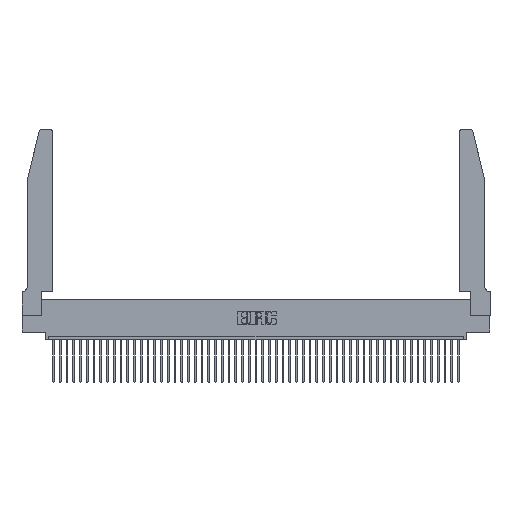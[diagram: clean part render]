
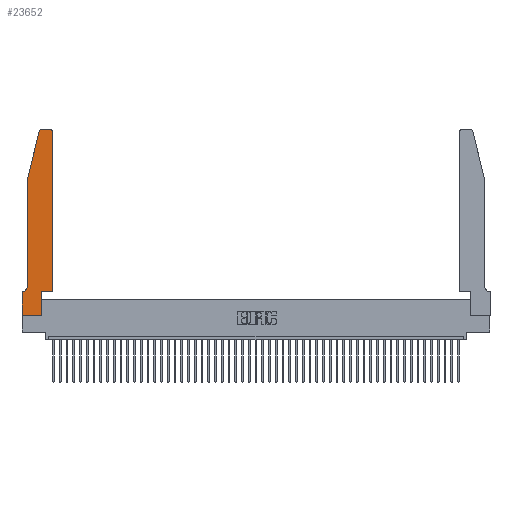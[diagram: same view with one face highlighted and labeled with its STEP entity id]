
A CAD part, top view. The second image highlights one B-rep face of the part: STEP entity #23652.
In plain terms, the highlighted planar face has unit normal (0, 0, 1).
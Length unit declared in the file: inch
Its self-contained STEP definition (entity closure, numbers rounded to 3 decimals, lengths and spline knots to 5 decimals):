
#334 = VERTEX_POINT ( 'NONE', #31678 ) ;
#384 = ORIENTED_EDGE ( 'NONE', *, *, #39325, .T. ) ;
#534 = VERTEX_POINT ( 'NONE', #18231 ) ;
#809 = VECTOR ( 'NONE', #45844, 39.37008 ) ;
#1754 = LINE ( 'NONE', #44460, #23940 ) ;
#2091 = CARTESIAN_POINT ( 'NONE',  ( 0.2605, 2.75, 0.37 ) ) ;
#2158 = CARTESIAN_POINT ( 'NONE',  ( 0.4505, 0.35, 0.37 ) ) ;
#2285 = VECTOR ( 'NONE', #21244, 39.37008 ) ;
#2481 = LINE ( 'NONE', #46527, #35197 ) ;
#2834 = EDGE_CURVE ( 'NONE', #21387, #24758, #18987, .T. ) ;
#3673 = AXIS2_PLACEMENT_3D ( 'NONE', #34987, #16286, #5398 ) ;
#5037 = EDGE_CURVE ( 'NONE', #47664, #334, #12817, .T. ) ;
#5147 = DIRECTION ( 'NONE',  ( 1., 0., 0. ) ) ;
#5398 = DIRECTION ( 'NONE',  ( 1., 0., 0. ) ) ;
#6125 = ORIENTED_EDGE ( 'NONE', *, *, #2834, .T. ) ;
#6896 = DIRECTION ( 'NONE',  ( 0., 1., 0. ) ) ;
#8666 = VECTOR ( 'NONE', #9770, 39.37008 ) ;
#9221 = CARTESIAN_POINT ( 'NONE',  ( 0.0755, 0.35, 0.37 ) ) ;
#9326 = PLANE ( 'NONE',  #3673 ) ;
#9512 = ORIENTED_EDGE ( 'NONE', *, *, #25258, .T. ) ;
#9770 = DIRECTION ( 'NONE',  ( -1., 0., 0. ) ) ;
#9812 = CARTESIAN_POINT ( 'NONE',  ( 0., 0., 0.37 ) ) ;
#10201 = VERTEX_POINT ( 'NONE', #44022 ) ;
#10292 = CARTESIAN_POINT ( 'NONE',  ( 0., 0., 0.37 ) ) ;
#10996 = VECTOR ( 'NONE', #5147, 39.37008 ) ;
#11121 = EDGE_CURVE ( 'NONE', #11462, #534, #1754, .T. ) ;
#11462 = VERTEX_POINT ( 'NONE', #35805 ) ;
#12066 = VERTEX_POINT ( 'NONE', #27359 ) ;
#12120 = EDGE_CURVE ( 'NONE', #534, #27906, #27299, .T. ) ;
#12140 = ORIENTED_EDGE ( 'NONE', *, *, #16140, .T. ) ;
#12817 = LINE ( 'NONE', #9812, #2285 ) ;
#12929 = CARTESIAN_POINT ( 'NONE',  ( 0.0755, 2., 0.37 ) ) ;
#13012 = CIRCLE ( 'NONE', #23377, 0.03 ) ;
#13439 = DIRECTION ( 'NONE',  ( 0., 1., 0. ) ) ;
#14076 = CARTESIAN_POINT ( 'NONE',  ( 0.0055, 0.35, 0.37 ) ) ;
#14097 = AXIS2_PLACEMENT_3D ( 'NONE', #31007, #34799, #16276 ) ;
#14625 = DIRECTION ( 'NONE',  ( 0., 0., 1. ) ) ;
#14657 = CARTESIAN_POINT ( 'NONE',  ( 0., 0.35, 0.37 ) ) ;
#14706 = DIRECTION ( 'NONE',  ( -0.239, -0.971, 0. ) ) ;
#14954 = EDGE_CURVE ( 'NONE', #40110, #21387, #40559, .T. ) ;
#16140 = EDGE_CURVE ( 'NONE', #24758, #47664, #36387, .T. ) ;
#16276 = DIRECTION ( 'NONE',  ( -1., 0., 0. ) ) ;
#16286 = DIRECTION ( 'NONE',  ( 0., 0., 1. ) ) ;
#16983 = DIRECTION ( 'NONE',  ( 0., 0., 1. ) ) ;
#17007 = VECTOR ( 'NONE', #45388, 39.37008 ) ;
#17959 = CARTESIAN_POINT ( 'NONE',  ( 0.0755, 2., 0.37 ) ) ;
#18231 = CARTESIAN_POINT ( 'NONE',  ( 0.2865, 0.35, 0.37 ) ) ;
#18987 = CIRCLE ( 'NONE', #14097, 0.07 ) ;
#19658 = CARTESIAN_POINT ( 'NONE',  ( 0.4505, 0.35, 0.37 ) ) ;
#21244 = DIRECTION ( 'NONE',  ( 0., -1., 0. ) ) ;
#21387 = VERTEX_POINT ( 'NONE', #24876 ) ;
#22283 = DIRECTION ( 'NONE',  ( 1., 0., 0. ) ) ;
#22894 = ORIENTED_EDGE ( 'NONE', *, *, #33640, .T. ) ;
#23377 = AXIS2_PLACEMENT_3D ( 'NONE', #34662, #16983, #24681 ) ;
#23652 = ADVANCED_FACE ( 'NONE', ( #28387 ), #9326, .T. ) ;
#23940 = VECTOR ( 'NONE', #6896, 39.37008 ) ;
#24477 = LINE ( 'NONE', #2091, #8666 ) ;
#24681 = DIRECTION ( 'NONE',  ( 1., 0., 0. ) ) ;
#24758 = VERTEX_POINT ( 'NONE', #14076 ) ;
#24876 = CARTESIAN_POINT ( 'NONE',  ( 0.0755, 0.42, 0.37 ) ) ;
#25055 = VERTEX_POINT ( 'NONE', #32780 ) ;
#25258 = EDGE_CURVE ( 'NONE', #25055, #44021, #13012, .T. ) ;
#27299 = LINE ( 'NONE', #19658, #10996 ) ;
#27308 = ORIENTED_EDGE ( 'NONE', *, *, #14954, .T. ) ;
#27359 = CARTESIAN_POINT ( 'NONE',  ( 0.25487, 2.72718, 0.37 ) ) ;
#27906 = VERTEX_POINT ( 'NONE', #2158 ) ;
#28387 = FACE_OUTER_BOUND ( 'NONE', #43216, .T. ) ;
#29068 = CARTESIAN_POINT ( 'NONE',  ( 0.4205, 2.75, 0.37 ) ) ;
#29402 = ORIENTED_EDGE ( 'NONE', *, *, #45147, .T. ) ;
#30463 = LINE ( 'NONE', #10292, #41052 ) ;
#30565 = EDGE_CURVE ( 'NONE', #27906, #25055, #2481, .T. ) ;
#30820 = AXIS2_PLACEMENT_3D ( 'NONE', #33434, #14625, #22283 ) ;
#31007 = CARTESIAN_POINT ( 'NONE',  ( 0.0055, 0.42, 0.37 ) ) ;
#31678 = CARTESIAN_POINT ( 'NONE',  ( 0., 0., 0.37 ) ) ;
#32780 = CARTESIAN_POINT ( 'NONE',  ( 0.4505, 2.72, 0.37 ) ) ;
#33269 = CIRCLE ( 'NONE', #30820, 0.03 ) ;
#33434 = CARTESIAN_POINT ( 'NONE',  ( 0.284, 2.72, 0.37 ) ) ;
#33640 = EDGE_CURVE ( 'NONE', #44021, #10201, #24477, .T. ) ;
#33672 = ORIENTED_EDGE ( 'NONE', *, *, #30565, .T. ) ;
#33988 = ORIENTED_EDGE ( 'NONE', *, *, #44829, .T. ) ;
#34662 = CARTESIAN_POINT ( 'NONE',  ( 0.4205, 2.72, 0.37 ) ) ;
#34799 = DIRECTION ( 'NONE',  ( 0., 0., -1. ) ) ;
#34987 = CARTESIAN_POINT ( 'NONE',  ( 0., 0.35, 0.37 ) ) ;
#35197 = VECTOR ( 'NONE', #13439, 39.37008 ) ;
#35266 = ORIENTED_EDGE ( 'NONE', *, *, #11121, .T. ) ;
#35787 = DIRECTION ( 'NONE',  ( 1., 0., 0. ) ) ;
#35805 = CARTESIAN_POINT ( 'NONE',  ( 0.2865, 0., 0.37 ) ) ;
#36387 = LINE ( 'NONE', #9221, #17007 ) ;
#36894 = ORIENTED_EDGE ( 'NONE', *, *, #5037, .T. ) ;
#39325 = EDGE_CURVE ( 'NONE', #334, #11462, #30463, .T. ) ;
#40110 = VERTEX_POINT ( 'NONE', #43679 ) ;
#40559 = LINE ( 'NONE', #12929, #809 ) ;
#41052 = VECTOR ( 'NONE', #35787, 39.37008 ) ;
#43094 = VECTOR ( 'NONE', #14706, 39.37008 ) ;
#43216 = EDGE_LOOP ( 'NONE', ( #22894, #33988, #29402, #27308, #6125, #12140, #36894, #384, #35266, #44967, #33672, #9512 ) ) ;
#43679 = CARTESIAN_POINT ( 'NONE',  ( 0.0755, 2., 0.37 ) ) ;
#44021 = VERTEX_POINT ( 'NONE', #29068 ) ;
#44022 = CARTESIAN_POINT ( 'NONE',  ( 0.284, 2.75, 0.37 ) ) ;
#44460 = CARTESIAN_POINT ( 'NONE',  ( 0.2865, 0.35, 0.37 ) ) ;
#44829 = EDGE_CURVE ( 'NONE', #10201, #12066, #33269, .T. ) ;
#44967 = ORIENTED_EDGE ( 'NONE', *, *, #12120, .T. ) ;
#45147 = EDGE_CURVE ( 'NONE', #12066, #40110, #46584, .T. ) ;
#45388 = DIRECTION ( 'NONE',  ( -1., 0., 0. ) ) ;
#45844 = DIRECTION ( 'NONE',  ( 0., -1., 0. ) ) ;
#46527 = CARTESIAN_POINT ( 'NONE',  ( 0.4505, 0.35, 0.37 ) ) ;
#46584 = LINE ( 'NONE', #17959, #43094 ) ;
#47664 = VERTEX_POINT ( 'NONE', #14657 ) ;
